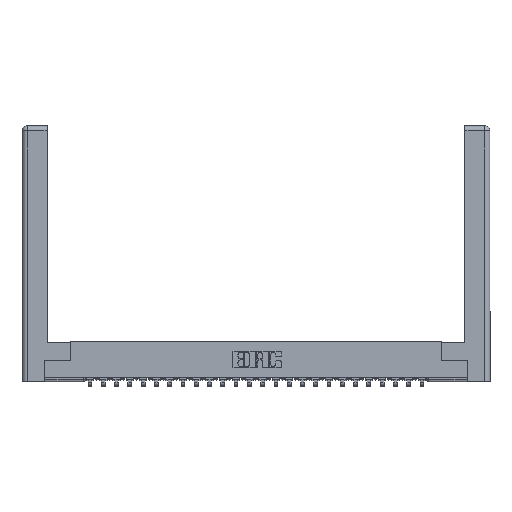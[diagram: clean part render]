
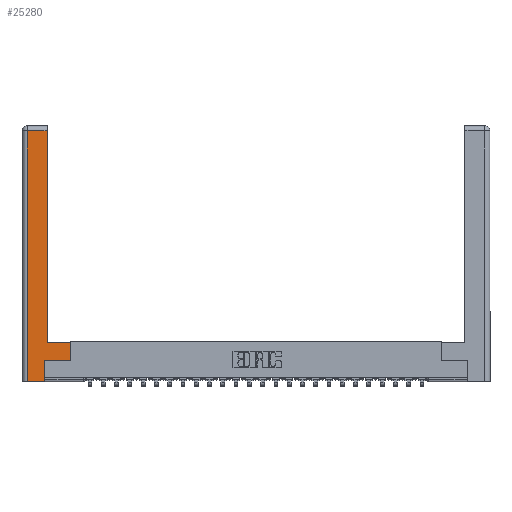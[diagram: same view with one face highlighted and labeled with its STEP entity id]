
A CAD part, top view. The second image highlights one B-rep face of the part: STEP entity #25280.
In plain terms, the highlighted planar face has unit normal (0, 0, 1).
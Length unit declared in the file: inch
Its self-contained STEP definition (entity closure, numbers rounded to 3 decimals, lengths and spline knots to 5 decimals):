
#389 = DIRECTION ( 'NONE',  ( 0., 1., 0. ) ) ;
#1201 = CARTESIAN_POINT ( 'NONE',  ( 0.265, 0.245, 0. ) ) ;
#1656 = DIRECTION ( 'NONE',  ( 1., 0., 0. ) ) ;
#2047 = CARTESIAN_POINT ( 'NONE',  ( 0.295, 0.45, 0. ) ) ;
#2237 = DIRECTION ( 'NONE',  ( 0., 0., -1. ) ) ;
#3002 = CARTESIAN_POINT ( 'NONE',  ( 0.0615, 2.94, 0. ) ) ;
#3599 = ORIENTED_EDGE ( 'NONE', *, *, #24469, .T. ) ;
#3777 = ORIENTED_EDGE ( 'NONE', *, *, #25074, .T. ) ;
#3927 = LINE ( 'NONE', #16703, #7903 ) ;
#5471 = VECTOR ( 'NONE', #26249, 39.37008 ) ;
#5691 = CARTESIAN_POINT ( 'NONE',  ( 0.295, 2.94, 0. ) ) ;
#6635 = AXIS2_PLACEMENT_3D ( 'NONE', #27704, #2237, #8478 ) ;
#6805 = LINE ( 'NONE', #24218, #5471 ) ;
#7254 = DIRECTION ( 'NONE',  ( -1., 0., 0. ) ) ;
#7386 = VECTOR ( 'NONE', #13673, 39.37008 ) ;
#7622 = ORIENTED_EDGE ( 'NONE', *, *, #27737, .T. ) ;
#7698 = VERTEX_POINT ( 'NONE', #18120 ) ;
#7903 = VECTOR ( 'NONE', #18899, 39.37008 ) ;
#8178 = VERTEX_POINT ( 'NONE', #5691 ) ;
#8478 = DIRECTION ( 'NONE',  ( -1., 0., 0. ) ) ;
#8577 = VERTEX_POINT ( 'NONE', #11186 ) ;
#9280 = VECTOR ( 'NONE', #389, 39.37008 ) ;
#11186 = CARTESIAN_POINT ( 'NONE',  ( 0.0615, 2.94, 0. ) ) ;
#12477 = VECTOR ( 'NONE', #7254, 39.37008 ) ;
#12662 = CARTESIAN_POINT ( 'NONE',  ( 0.0615, 0., 0. ) ) ;
#13028 = CARTESIAN_POINT ( 'NONE',  ( 0.265, 0.245, 0. ) ) ;
#13053 = VERTEX_POINT ( 'NONE', #20741 ) ;
#13673 = DIRECTION ( 'NONE',  ( 0., 1., 0. ) ) ;
#14124 = ORIENTED_EDGE ( 'NONE', *, *, #23704, .T. ) ;
#15019 = LINE ( 'NONE', #17807, #9280 ) ;
#15306 = VERTEX_POINT ( 'NONE', #17799 ) ;
#15815 = EDGE_LOOP ( 'NONE', ( #21429, #14124, #27716, #3599, #23069, #7622, #22802, #3777 ) ) ;
#16163 = VERTEX_POINT ( 'NONE', #1201 ) ;
#16703 = CARTESIAN_POINT ( 'NONE',  ( 0.0615, 0., 0. ) ) ;
#16827 = PLANE ( 'NONE',  #6635 ) ;
#16898 = DIRECTION ( 'NONE',  ( 1., 0., 0. ) ) ;
#16986 = CARTESIAN_POINT ( 'NONE',  ( 0.565, 0.245, 0. ) ) ;
#17110 = LINE ( 'NONE', #2047, #24505 ) ;
#17615 = EDGE_CURVE ( 'NONE', #8577, #17621, #3927, .T. ) ;
#17621 = VERTEX_POINT ( 'NONE', #12662 ) ;
#17799 = CARTESIAN_POINT ( 'NONE',  ( 0.565, 0.245, 0. ) ) ;
#17807 = CARTESIAN_POINT ( 'NONE',  ( 0.565, 0.45, 0. ) ) ;
#17925 = VERTEX_POINT ( 'NONE', #22550 ) ;
#18120 = CARTESIAN_POINT ( 'NONE',  ( 0.295, 0.45, 0. ) ) ;
#18841 = LINE ( 'NONE', #13028, #7386 ) ;
#18899 = DIRECTION ( 'NONE',  ( 0., -1., 0. ) ) ;
#20035 = EDGE_CURVE ( 'NONE', #7698, #8178, #6805, .T. ) ;
#20139 = FACE_OUTER_BOUND ( 'NONE', #15815, .T. ) ;
#20741 = CARTESIAN_POINT ( 'NONE',  ( 0.265, 0., 0. ) ) ;
#21429 = ORIENTED_EDGE ( 'NONE', *, *, #20035, .T. ) ;
#21883 = VECTOR ( 'NONE', #1656, 39.37008 ) ;
#22276 = VECTOR ( 'NONE', #16898, 39.37008 ) ;
#22550 = CARTESIAN_POINT ( 'NONE',  ( 0.565, 0.45, 0. ) ) ;
#22802 = ORIENTED_EDGE ( 'NONE', *, *, #25985, .T. ) ;
#23069 = ORIENTED_EDGE ( 'NONE', *, *, #24791, .T. ) ;
#23704 = EDGE_CURVE ( 'NONE', #8178, #8577, #25591, .T. ) ;
#23930 = LINE ( 'NONE', #16986, #22276 ) ;
#24218 = CARTESIAN_POINT ( 'NONE',  ( 0.295, 3., 0. ) ) ;
#24469 = EDGE_CURVE ( 'NONE', #17621, #13053, #27545, .T. ) ;
#24505 = VECTOR ( 'NONE', #25457, 39.37008 ) ;
#24791 = EDGE_CURVE ( 'NONE', #13053, #16163, #18841, .T. ) ;
#25074 = EDGE_CURVE ( 'NONE', #17925, #7698, #17110, .T. ) ;
#25280 = ADVANCED_FACE ( 'NONE', ( #20139 ), #16827, .F. ) ;
#25457 = DIRECTION ( 'NONE',  ( -1., 0., 0. ) ) ;
#25591 = LINE ( 'NONE', #3002, #12477 ) ;
#25985 = EDGE_CURVE ( 'NONE', #15306, #17925, #15019, .T. ) ;
#26249 = DIRECTION ( 'NONE',  ( 0., 1., 0. ) ) ;
#27290 = CARTESIAN_POINT ( 'NONE',  ( 0.265, 0., 0. ) ) ;
#27545 = LINE ( 'NONE', #27290, #21883 ) ;
#27704 = CARTESIAN_POINT ( 'NONE',  ( 0., 0., 0. ) ) ;
#27716 = ORIENTED_EDGE ( 'NONE', *, *, #17615, .T. ) ;
#27737 = EDGE_CURVE ( 'NONE', #16163, #15306, #23930, .T. ) ;
